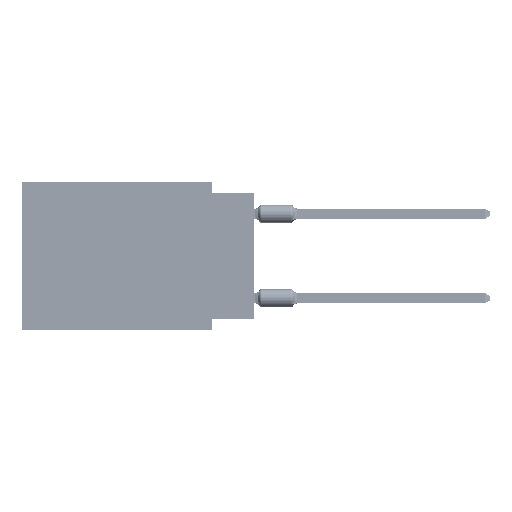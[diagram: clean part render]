
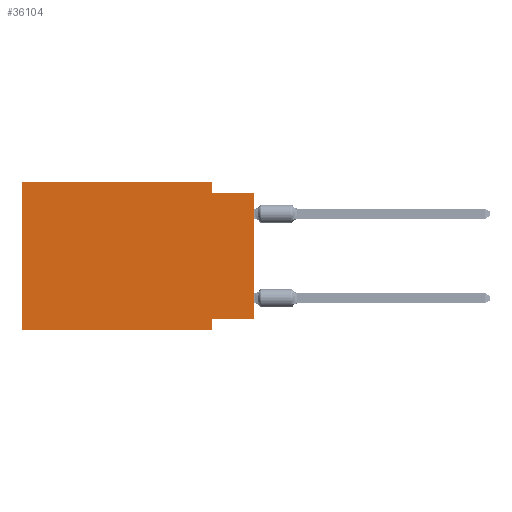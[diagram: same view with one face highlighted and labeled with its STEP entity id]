
A CAD part, left-side view. The second image highlights one B-rep face of the part: STEP entity #36104.
In plain terms, the highlighted planar face has unit normal (-1, 0, 0).
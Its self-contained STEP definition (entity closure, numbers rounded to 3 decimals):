
#736 = VERTEX_POINT ( 'NONE', #11080 ) ;
#1942 = ORIENTED_EDGE ( 'NONE', *, *, #12322, .F. ) ;
#3520 = FACE_OUTER_BOUND ( 'NONE', #18819, .T. ) ;
#3839 = CARTESIAN_POINT ( 'NONE',  ( 0., 0., -8.255 ) ) ;
#5016 = DIRECTION ( 'NONE',  ( 1., 0., 0. ) ) ;
#5162 = EDGE_CURVE ( 'NONE', #63708, #30725, #39952, .T. ) ;
#9161 = ORIENTED_EDGE ( 'NONE', *, *, #69952, .F. ) ;
#10662 = LINE ( 'NONE', #57536, #19107 ) ;
#11080 = CARTESIAN_POINT ( 'NONE',  ( 0., 2.54, 0. ) ) ;
#11700 = CARTESIAN_POINT ( 'NONE',  ( 0., 13.97, -8.89 ) ) ;
#12322 = EDGE_CURVE ( 'NONE', #30725, #736, #44662, .T. ) ;
#13335 = VECTOR ( 'NONE', #54792, 1000. ) ;
#13747 = LINE ( 'NONE', #19839, #31575 ) ;
#14008 = LINE ( 'NONE', #31550, #13335 ) ;
#15035 = ORIENTED_EDGE ( 'NONE', *, *, #16208, .T. ) ;
#16208 = EDGE_CURVE ( 'NONE', #45522, #29888, #14008, .T. ) ;
#16322 = CARTESIAN_POINT ( 'NONE',  ( 0., 13.97, 0. ) ) ;
#18819 = EDGE_LOOP ( 'NONE', ( #15035, #56316, #9161, #1942, #22902, #28279, #33090, #67647 ) ) ;
#19107 = VECTOR ( 'NONE', #57162, 1000. ) ;
#19747 = CARTESIAN_POINT ( 'NONE',  ( 0., 2.54, -8.89 ) ) ;
#19839 = CARTESIAN_POINT ( 'NONE',  ( 0., 0., -8.255 ) ) ;
#20198 = EDGE_CURVE ( 'NONE', #38783, #35112, #37098, .T. ) ;
#21981 = VECTOR ( 'NONE', #42933, 1000. ) ;
#22186 = PLANE ( 'NONE',  #28076 ) ;
#22902 = ORIENTED_EDGE ( 'NONE', *, *, #5162, .F. ) ;
#25174 = CARTESIAN_POINT ( 'NONE',  ( 0., 0., -0.635 ) ) ;
#25389 = LINE ( 'NONE', #71885, #21981 ) ;
#28076 = AXIS2_PLACEMENT_3D ( 'NONE', #61817, #5016, #56498 ) ;
#28279 = ORIENTED_EDGE ( 'NONE', *, *, #72421, .T. ) ;
#29093 = LINE ( 'NONE', #52341, #54702 ) ;
#29888 = VERTEX_POINT ( 'NONE', #25174 ) ;
#30725 = VERTEX_POINT ( 'NONE', #48246 ) ;
#31550 = CARTESIAN_POINT ( 'NONE',  ( 0., 0., 0. ) ) ;
#31575 = VECTOR ( 'NONE', #41596, 1000. ) ;
#33001 = VERTEX_POINT ( 'NONE', #59174 ) ;
#33090 = ORIENTED_EDGE ( 'NONE', *, *, #20198, .F. ) ;
#35112 = VERTEX_POINT ( 'NONE', #19747 ) ;
#36005 = CARTESIAN_POINT ( 'NONE',  ( 0., 2.54, -8.255 ) ) ;
#36104 = ADVANCED_FACE ( 'NONE', ( #3520 ), #22186, .F. ) ;
#37098 = LINE ( 'NONE', #66055, #39313 ) ;
#37365 = EDGE_CURVE ( 'NONE', #33001, #29888, #25389, .T. ) ;
#38783 = VERTEX_POINT ( 'NONE', #36005 ) ;
#38955 = CARTESIAN_POINT ( 'NONE',  ( 0., 13.97, 0. ) ) ;
#39313 = VECTOR ( 'NONE', #72135, 1000. ) ;
#39952 = LINE ( 'NONE', #16322, #51737 ) ;
#41596 = DIRECTION ( 'NONE',  ( 0., 1., 0. ) ) ;
#42933 = DIRECTION ( 'NONE',  ( 0., -1., 0. ) ) ;
#44662 = LINE ( 'NONE', #38955, #71272 ) ;
#45522 = VERTEX_POINT ( 'NONE', #3839 ) ;
#46631 = DIRECTION ( 'NONE',  ( 0., -1., 0. ) ) ;
#48246 = CARTESIAN_POINT ( 'NONE',  ( 0., 13.97, 0. ) ) ;
#51737 = VECTOR ( 'NONE', #73496, 1000. ) ;
#52341 = CARTESIAN_POINT ( 'NONE',  ( 0., 13.97, -8.89 ) ) ;
#54702 = VECTOR ( 'NONE', #46631, 1000. ) ;
#54792 = DIRECTION ( 'NONE',  ( 0., 0., 1. ) ) ;
#56316 = ORIENTED_EDGE ( 'NONE', *, *, #37365, .F. ) ;
#56498 = DIRECTION ( 'NONE',  ( 0., 0., -1. ) ) ;
#57162 = DIRECTION ( 'NONE',  ( 0., 0., -1. ) ) ;
#57536 = CARTESIAN_POINT ( 'NONE',  ( 0., 2.54, 0. ) ) ;
#59174 = CARTESIAN_POINT ( 'NONE',  ( 0., 2.54, -0.635 ) ) ;
#61793 = DIRECTION ( 'NONE',  ( 0., -1., 0. ) ) ;
#61817 = CARTESIAN_POINT ( 'NONE',  ( 0., 13.97, 0. ) ) ;
#63708 = VERTEX_POINT ( 'NONE', #11700 ) ;
#66055 = CARTESIAN_POINT ( 'NONE',  ( 0., 2.54, -8.89 ) ) ;
#67647 = ORIENTED_EDGE ( 'NONE', *, *, #74286, .F. ) ;
#69952 = EDGE_CURVE ( 'NONE', #736, #33001, #10662, .T. ) ;
#71272 = VECTOR ( 'NONE', #61793, 1000. ) ;
#71885 = CARTESIAN_POINT ( 'NONE',  ( 0., 0., -0.635 ) ) ;
#72135 = DIRECTION ( 'NONE',  ( 0., 0., -1. ) ) ;
#72421 = EDGE_CURVE ( 'NONE', #63708, #35112, #29093, .T. ) ;
#73496 = DIRECTION ( 'NONE',  ( 0., 0., 1. ) ) ;
#74286 = EDGE_CURVE ( 'NONE', #45522, #38783, #13747, .T. ) ;
